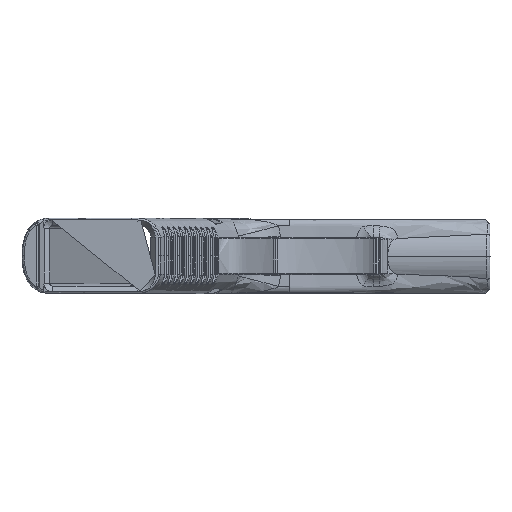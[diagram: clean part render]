
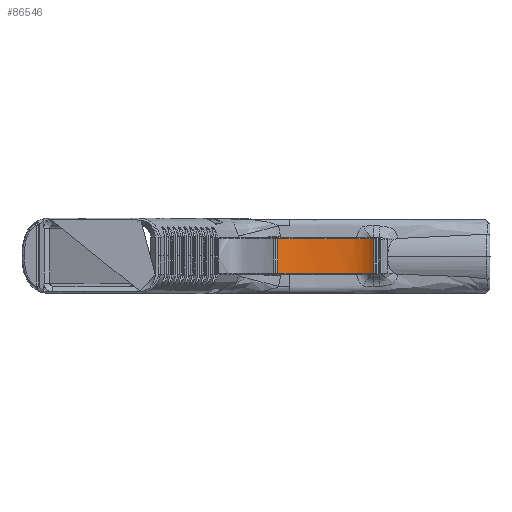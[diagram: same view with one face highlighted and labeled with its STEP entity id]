
A CAD part, top view. The second image highlights one B-rep face of the part: STEP entity #86546.
In plain terms, the highlighted free-form (B-spline) face has degree [3, 1] with [6, 2] control points.
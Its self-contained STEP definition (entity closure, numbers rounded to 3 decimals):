
#3228 = VERTEX_POINT ( 'NONE', #298531 ) ;
#7095 = CARTESIAN_POINT ( 'NONE',  ( 109.72, -5.842, -57.351 ) ) ;
#7836 = VERTEX_POINT ( 'NONE', #362684 ) ;
#8367 = CARTESIAN_POINT ( 'NONE',  ( 118.339, -5.842, -57.616 ) ) ;
#14908 = FACE_OUTER_BOUND ( 'NONE', #35106, .T. ) ;
#17602 = CARTESIAN_POINT ( 'NONE',  ( 126.962, 5.842, -57.119 ) ) ;
#18870 = CARTESIAN_POINT ( 'NONE',  ( 134.23, 5.842, -54.64 ) ) ;
#20166 = CARTESIAN_POINT ( 'NONE',  ( 135.323, 5.842, -53.8 ) ) ;
#35106 = EDGE_LOOP ( 'NONE', ( #209837, #227409, #89637, #353460 ) ) ;
#36771 = CARTESIAN_POINT ( 'NONE',  ( 124.104, -5.842, -57.408 ) ) ;
#41748 = VECTOR ( 'NONE', #53226, 1000. ) ;
#45574 = CARTESIAN_POINT ( 'NONE',  ( 135.323, -5.842, -53.8 ) ) ;
#47280 = CARTESIAN_POINT ( 'NONE',  ( 116.165, 5.842, -57.634 ) ) ;
#49104 = DIRECTION ( 'NONE',  ( 0., 1., 0. ) ) ;
#52605 = VERTEX_POINT ( 'NONE', #177510 ) ;
#53226 = DIRECTION ( 'NONE',  ( 0., -1., 0. ) ) ;
#61749 = CARTESIAN_POINT ( 'NONE',  ( 126.057, -18.407, -57.504 ) ) ;
#64300 = CARTESIAN_POINT ( 'NONE',  ( 135.323, -18.407, -53.8 ) ) ;
#68530 = VERTEX_POINT ( 'NONE', #365585 ) ;
#71491 = CARTESIAN_POINT ( 'NONE',  ( 126.962, -5.842, -57.119 ) ) ;
#78220 = CARTESIAN_POINT ( 'NONE',  ( 107.607, 5.842, -57.006 ) ) ;
#79508 = CARTESIAN_POINT ( 'NONE',  ( 134.794, 5.842, -54.243 ) ) ;
#80063 = CARTESIAN_POINT ( 'NONE',  ( 102.348, 0., -55.098 ) ) ;
#86546 = ADVANCED_FACE ( 'NONE', ( #14908 ), #381670, .F. ) ;
#89637 = ORIENTED_EDGE ( 'NONE', *, *, #353911, .F. ) ;
#91446 = CARTESIAN_POINT ( 'NONE',  ( 106.968, -18.407, -57.633 ) ) ;
#97424 = CARTESIAN_POINT ( 'NONE',  ( 124.821, -5.842, -57.352 ) ) ;
#101230 = CARTESIAN_POINT ( 'NONE',  ( 111.849, -5.842, -57.565 ) ) ;
#105413 = CARTESIAN_POINT ( 'NONE',  ( 104.873, 5.842, -56.285 ) ) ;
#124928 = CARTESIAN_POINT ( 'NONE',  ( 132.341, 5.842, -56.299 ) ) ;
#127144 = CARTESIAN_POINT ( 'NONE',  ( 126.25, -5.842, -57.208 ) ) ;
#133067 = EDGE_CURVE ( 'NONE', #52605, #3228, #295613, .T. ) ;
#135082 = CARTESIAN_POINT ( 'NONE',  ( 124.104, 5.842, -57.408 ) ) ;
#136363 = CARTESIAN_POINT ( 'NONE',  ( 109.013, 5.842, -57.256 ) ) ;
#137657 = CARTESIAN_POINT ( 'NONE',  ( 111.849, 5.842, -57.565 ) ) ;
#148848 = B_SPLINE_CURVE_WITH_KNOTS ( 'NONE', 3,
 ( #45574, #295616, #218715, #348129, #260385, #333847, #304237, #71491, #127144, #97424, #36771, #364841, #244818, #8367, #185323, #218857, #217595, #158144, #101230, #7095, #243535, #154342, #362298, #361027, #273241, #156873 ),
 .UNSPECIFIED., .F., .F.,
 ( 4, 2, 2, 2, 2, 2, 2, 2, 2, 2, 2, 2, 4 ),
 ( 0., 0.063, 0.125, 0.25, 0.313, 0.375, 0.5, 0.563, 0.625, 0.75, 0.813, 0.875, 1. ),
 .UNSPECIFIED. ) ;
#154342 = CARTESIAN_POINT ( 'NONE',  ( 107.607, -5.842, -57.006 ) ) ;
#156873 = CARTESIAN_POINT ( 'NONE',  ( 102.348, -5.842, -55.098 ) ) ;
#158144 = CARTESIAN_POINT ( 'NONE',  ( 113.281, -5.842, -57.616 ) ) ;
#166147 = CARTESIAN_POINT ( 'NONE',  ( 126.25, 5.842, -57.208 ) ) ;
#167427 = CARTESIAN_POINT ( 'NONE',  ( 115.442, 5.842, -57.637 ) ) ;
#168720 = CARTESIAN_POINT ( 'NONE',  ( 109.72, 5.842, -57.351 ) ) ;
#177510 = CARTESIAN_POINT ( 'NONE',  ( 102.348, 5.842, -55.098 ) ) ;
#183166 = CARTESIAN_POINT ( 'NONE',  ( 135.323, 5.842, -53.8 ) ) ;
#185323 = CARTESIAN_POINT ( 'NONE',  ( 117.614, -5.842, -57.623 ) ) ;
#194176 = VECTOR ( 'NONE', #49104, 1000. ) ;
#195865 = CARTESIAN_POINT ( 'NONE',  ( 132.394, 5.842, -55.655 ) ) ;
#197151 = CARTESIAN_POINT ( 'NONE',  ( 133.033, 5.842, -55.345 ) ) ;
#198711 = LINE ( 'NONE', #80063, #194176 ) ;
#198905 = EDGE_CURVE ( 'NONE', #68530, #52605, #198711, .T. ) ;
#209071 = CARTESIAN_POINT ( 'NONE',  ( 114.743, -18.407, -57.686 ) ) ;
#209837 = ORIENTED_EDGE ( 'NONE', *, *, #198905, .F. ) ;
#217595 = CARTESIAN_POINT ( 'NONE',  ( 115.442, -5.842, -57.637 ) ) ;
#218715 = CARTESIAN_POINT ( 'NONE',  ( 134.23, -5.842, -54.64 ) ) ;
#218857 = CARTESIAN_POINT ( 'NONE',  ( 116.165, -5.842, -57.634 ) ) ;
#222077 = EDGE_CURVE ( 'NONE', #7836, #68530, #148848, .T. ) ;
#224297 = CARTESIAN_POINT ( 'NONE',  ( 129.072, 5.842, -56.772 ) ) ;
#225594 = CARTESIAN_POINT ( 'NONE',  ( 103.577, 5.842, -55.772 ) ) ;
#226871 = CARTESIAN_POINT ( 'NONE',  ( 121.95, 5.842, -57.541 ) ) ;
#227409 = ORIENTED_EDGE ( 'NONE', *, *, #222077, .F. ) ;
#243535 = CARTESIAN_POINT ( 'NONE',  ( 109.013, -5.842, -57.256 ) ) ;
#244818 = CARTESIAN_POINT ( 'NONE',  ( 120.508, -5.842, -57.583 ) ) ;
#256644 = CARTESIAN_POINT ( 'NONE',  ( 124.821, 5.842, -57.352 ) ) ;
#260385 = CARTESIAN_POINT ( 'NONE',  ( 132.394, -5.842, -55.655 ) ) ;
#272338 = CARTESIAN_POINT ( 'NONE',  ( 106.968, 5.842, -57.633 ) ) ;
#273241 = CARTESIAN_POINT ( 'NONE',  ( 103.577, -5.842, -55.772 ) ) ;
#282454 = CARTESIAN_POINT ( 'NONE',  ( 102.348, 5.842, -55.098 ) ) ;
#295613 = B_SPLINE_CURVE_WITH_KNOTS ( 'NONE', 3,
 ( #282454, #225594, #105413, #375388, #78220, #136363, #168720, #137657, #344390, #167427, #47280, #374101, #312169, #316014, #226871, #135082, #256644, #166147, #17602, #224297, #341817, #195865, #197151, #18870, #79508, #20166 ),
 .UNSPECIFIED., .F., .F.,
 ( 4, 2, 2, 2, 2, 2, 2, 2, 2, 2, 2, 2, 4 ),
 ( 0., 0.125, 0.188, 0.25, 0.375, 0.438, 0.5, 0.625, 0.688, 0.75, 0.875, 0.938, 1. ),
 .UNSPECIFIED. ) ;
#295616 = CARTESIAN_POINT ( 'NONE',  ( 134.794, -5.842, -54.243 ) ) ;
#296979 = CARTESIAN_POINT ( 'NONE',  ( 126.057, 5.842, -57.504 ) ) ;
#298531 = CARTESIAN_POINT ( 'NONE',  ( 135.323, 5.842, -53.8 ) ) ;
#299528 = CARTESIAN_POINT ( 'NONE',  ( 102.348, 5.842, -55.098 ) ) ;
#304237 = CARTESIAN_POINT ( 'NONE',  ( 129.072, -5.842, -56.772 ) ) ;
#312169 = CARTESIAN_POINT ( 'NONE',  ( 118.339, 5.842, -57.616 ) ) ;
#316014 = CARTESIAN_POINT ( 'NONE',  ( 120.508, 5.842, -57.583 ) ) ;
#321923 = CARTESIAN_POINT ( 'NONE',  ( 135.323, -6.282, -53.8 ) ) ;
#327899 = CARTESIAN_POINT ( 'NONE',  ( 102.348, -18.407, -55.098 ) ) ;
#333847 = CARTESIAN_POINT ( 'NONE',  ( 130.438, -5.842, -56.436 ) ) ;
#337541 = LINE ( 'NONE', #321923, #41748 ) ;
#341817 = CARTESIAN_POINT ( 'NONE',  ( 130.438, 5.842, -56.436 ) ) ;
#344390 = CARTESIAN_POINT ( 'NONE',  ( 113.281, 5.842, -57.616 ) ) ;
#348129 = CARTESIAN_POINT ( 'NONE',  ( 133.033, -5.842, -55.345 ) ) ;
#353460 = ORIENTED_EDGE ( 'NONE', *, *, #133067, .F. ) ;
#353911 = EDGE_CURVE ( 'NONE', #3228, #7836, #337541, .T. ) ;
#360137 = CARTESIAN_POINT ( 'NONE',  ( 132.341, -18.407, -56.299 ) ) ;
#361027 = CARTESIAN_POINT ( 'NONE',  ( 104.873, -5.842, -56.285 ) ) ;
#361381 = CARTESIAN_POINT ( 'NONE',  ( 114.743, 5.842, -57.686 ) ) ;
#362298 = CARTESIAN_POINT ( 'NONE',  ( 106.91, -5.842, -56.851 ) ) ;
#362684 = CARTESIAN_POINT ( 'NONE',  ( 135.323, -5.842, -53.8 ) ) ;
#364841 = CARTESIAN_POINT ( 'NONE',  ( 121.95, -5.842, -57.541 ) ) ;
#365585 = CARTESIAN_POINT ( 'NONE',  ( 102.348, -5.842, -55.098 ) ) ;
#374101 = CARTESIAN_POINT ( 'NONE',  ( 117.614, 5.842, -57.623 ) ) ;
#375388 = CARTESIAN_POINT ( 'NONE',  ( 106.91, 5.842, -56.851 ) ) ;
#381670 = B_SPLINE_SURFACE_WITH_KNOTS ( 'NONE', 3, 1, ( 
 ( #299528, #327899 ),
 ( #272338, #91446 ),
 ( #361381, #209071 ),
 ( #296979, #61749 ),
 ( #124928, #360137 ),
 ( #183166, #64300 ) ),
 .UNSPECIFIED., .F., .F., .F.,
 ( 4, 1, 1, 4 ),
 ( 2, 2 ),
 ( 0.023, 0.453, 0.671, 0.984 ),
 ( 0., 2.425 ),
 .UNSPECIFIED. ) ;
